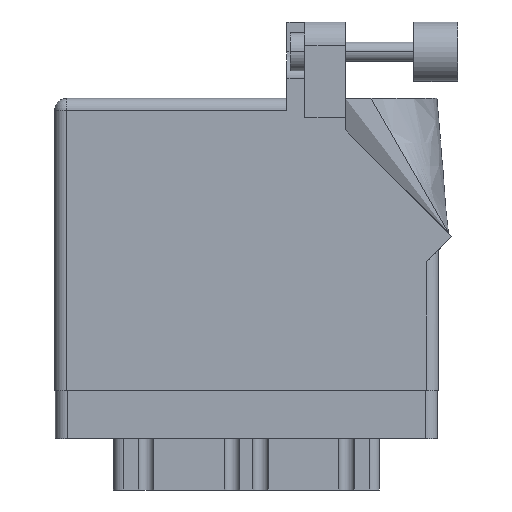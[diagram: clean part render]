
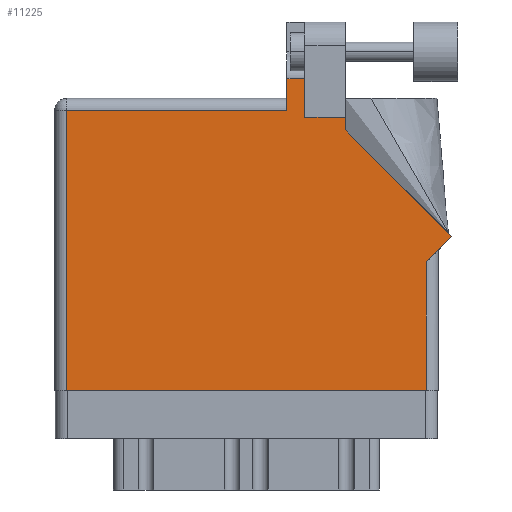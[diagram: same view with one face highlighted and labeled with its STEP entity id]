
A CAD part, front view. The second image highlights one B-rep face of the part: STEP entity #11225.
In plain terms, the highlighted face is planar.
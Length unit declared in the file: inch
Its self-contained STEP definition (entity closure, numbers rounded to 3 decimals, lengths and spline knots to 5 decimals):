
#45 = EDGE_CURVE ( 'NONE', #4962, #10918, #9773, .T. ) ;
#49 = CARTESIAN_POINT ( 'NONE',  ( 1.217, 1.6315, 0. ) ) ;
#969 = LINE ( 'NONE', #33979, #7254 ) ;
#1072 = CARTESIAN_POINT ( 'NONE',  ( 1.217, 1.53, 0. ) ) ;
#1214 = VERTEX_POINT ( 'NONE', #5678 ) ;
#1760 = VERTEX_POINT ( 'NONE', #22241 ) ;
#2330 = VECTOR ( 'NONE', #30479, 39.37008 ) ;
#2416 = VECTOR ( 'NONE', #27783, 39.37008 ) ;
#3102 = LINE ( 'NONE', #29622, #27266 ) ;
#3368 = CARTESIAN_POINT ( 'NONE',  ( 1.524, 1.43, 0. ) ) ;
#4962 = VERTEX_POINT ( 'NONE', #49 ) ;
#5392 = CARTESIAN_POINT ( 'NONE',  ( 1.311, 1.6315, 0. ) ) ;
#5678 = CARTESIAN_POINT ( 'NONE',  ( 1.948, 0.675, 0. ) ) ;
#6646 = EDGE_CURVE ( 'NONE', #15269, #12626, #13773, .T. ) ;
#7254 = VECTOR ( 'NONE', #25110, 39.37008 ) ;
#7283 = CARTESIAN_POINT ( 'NONE',  ( 0., 1.468, 0. ) ) ;
#7368 = VECTOR ( 'NONE', #35777, 39.37008 ) ;
#7680 = LINE ( 'NONE', #7283, #33889 ) ;
#7797 = DIRECTION ( 'NONE',  ( -1., 0., 0. ) ) ;
#7816 = DIRECTION ( 'NONE',  ( 0., 1., 0. ) ) ;
#8453 = VECTOR ( 'NONE', #7816, 39.37008 ) ;
#8519 = LINE ( 'NONE', #21163, #10813 ) ;
#9773 = LINE ( 'NONE', #1072, #2416 ) ;
#10010 = VECTOR ( 'NONE', #32989, 39.37008 ) ;
#10099 = EDGE_CURVE ( 'NONE', #18608, #1214, #24042, .T. ) ;
#10482 = AXIS2_PLACEMENT_3D ( 'NONE', #13750, #14530, #7797 ) ;
#10813 = VECTOR ( 'NONE', #23739, 39.37008 ) ;
#10918 = VERTEX_POINT ( 'NONE', #35880 ) ;
#11225 = ADVANCED_FACE ( 'NONE', ( #35449 ), #22645, .F. ) ;
#11258 = VECTOR ( 'NONE', #38801, 39.37008 ) ;
#11544 = EDGE_LOOP ( 'NONE', ( #30984, #26081, #30827, #28500, #20533, #27481, #18279, #28462, #35621, #21153, #14985 ) ) ;
#12437 = CARTESIAN_POINT ( 'NONE',  ( 1.524, 1.36442, 0. ) ) ;
#12626 = VERTEX_POINT ( 'NONE', #18458 ) ;
#12640 = EDGE_CURVE ( 'NONE', #22661, #18608, #17687, .T. ) ;
#13436 = DIRECTION ( 'NONE',  ( -1., 0., 0. ) ) ;
#13750 = CARTESIAN_POINT ( 'NONE',  ( 0., 1.53, 0. ) ) ;
#13773 = LINE ( 'NONE', #25844, #8453 ) ;
#14530 = DIRECTION ( 'NONE',  ( 0., 0., -1. ) ) ;
#14985 = ORIENTED_EDGE ( 'NONE', *, *, #28324, .T. ) ;
#15187 = DIRECTION ( 'NONE',  ( 0.707, 0.707, 0. ) ) ;
#15269 = VERTEX_POINT ( 'NONE', #12437 ) ;
#17625 = LINE ( 'NONE', #26726, #7368 ) ;
#17687 = LINE ( 'NONE', #18267, #11258 ) ;
#18267 = CARTESIAN_POINT ( 'NONE',  ( 0., 0., 0. ) ) ;
#18279 = ORIENTED_EDGE ( 'NONE', *, *, #10099, .T. ) ;
#18458 = CARTESIAN_POINT ( 'NONE',  ( 1.524, 1.43, 0. ) ) ;
#18608 = VERTEX_POINT ( 'NONE', #37759 ) ;
#19202 = LINE ( 'NONE', #3368, #2330 ) ;
#19732 = EDGE_CURVE ( 'NONE', #1214, #1760, #3102, .T. ) ;
#20533 = ORIENTED_EDGE ( 'NONE', *, *, #34644, .T. ) ;
#21153 = ORIENTED_EDGE ( 'NONE', *, *, #6646, .T. ) ;
#21163 = CARTESIAN_POINT ( 'NONE',  ( 0.062, 0., 0. ) ) ;
#22241 = CARTESIAN_POINT ( 'NONE',  ( 2.08071, 0.80771, 0. ) ) ;
#22645 = PLANE ( 'NONE',  #10482 ) ;
#22661 = VERTEX_POINT ( 'NONE', #27908 ) ;
#23739 = DIRECTION ( 'NONE',  ( 0., -1., 0. ) ) ;
#24042 = LINE ( 'NONE', #36070, #25377 ) ;
#25026 = VERTEX_POINT ( 'NONE', #28873 ) ;
#25110 = DIRECTION ( 'NONE',  ( -0.707, 0.707, 0. ) ) ;
#25377 = VECTOR ( 'NONE', #27594, 39.37008 ) ;
#25844 = CARTESIAN_POINT ( 'NONE',  ( 1.524, 1.36442, 0. ) ) ;
#26081 = ORIENTED_EDGE ( 'NONE', *, *, #35773, .T. ) ;
#26388 = VERTEX_POINT ( 'NONE', #31179 ) ;
#26726 = CARTESIAN_POINT ( 'NONE',  ( 1.64177, 1.6315, 0. ) ) ;
#27266 = VECTOR ( 'NONE', #15187, 39.37008 ) ;
#27481 = ORIENTED_EDGE ( 'NONE', *, *, #12640, .T. ) ;
#27594 = DIRECTION ( 'NONE',  ( 0., 1., 0. ) ) ;
#27783 = DIRECTION ( 'NONE',  ( 0., -1., 0. ) ) ;
#27908 = CARTESIAN_POINT ( 'NONE',  ( 0.062, 0., 0. ) ) ;
#28324 = EDGE_CURVE ( 'NONE', #12626, #26388, #19202, .T. ) ;
#28462 = ORIENTED_EDGE ( 'NONE', *, *, #19732, .T. ) ;
#28500 = ORIENTED_EDGE ( 'NONE', *, *, #31473, .T. ) ;
#28873 = CARTESIAN_POINT ( 'NONE',  ( 0.062, 1.468, 0. ) ) ;
#29298 = EDGE_CURVE ( 'NONE', #1760, #15269, #969, .T. ) ;
#29622 = CARTESIAN_POINT ( 'NONE',  ( 2.01, 0.737, 0. ) ) ;
#30231 = LINE ( 'NONE', #33378, #10010 ) ;
#30479 = DIRECTION ( 'NONE',  ( -1., 0., 0. ) ) ;
#30827 = ORIENTED_EDGE ( 'NONE', *, *, #45, .T. ) ;
#30984 = ORIENTED_EDGE ( 'NONE', *, *, #37310, .T. ) ;
#31179 = CARTESIAN_POINT ( 'NONE',  ( 1.311, 1.43, 0. ) ) ;
#31473 = EDGE_CURVE ( 'NONE', #10918, #25026, #7680, .T. ) ;
#32989 = DIRECTION ( 'NONE',  ( 0., 1., 0. ) ) ;
#33378 = CARTESIAN_POINT ( 'NONE',  ( 1.311, 1.43, 0. ) ) ;
#33889 = VECTOR ( 'NONE', #13436, 39.37008 ) ;
#33979 = CARTESIAN_POINT ( 'NONE',  ( 2.08071, 0.80771, 0. ) ) ;
#34644 = EDGE_CURVE ( 'NONE', #25026, #22661, #8519, .T. ) ;
#35282 = VERTEX_POINT ( 'NONE', #5392 ) ;
#35449 = FACE_OUTER_BOUND ( 'NONE', #11544, .T. ) ;
#35621 = ORIENTED_EDGE ( 'NONE', *, *, #29298, .T. ) ;
#35773 = EDGE_CURVE ( 'NONE', #35282, #4962, #17625, .T. ) ;
#35777 = DIRECTION ( 'NONE',  ( -1., 0., 0. ) ) ;
#35880 = CARTESIAN_POINT ( 'NONE',  ( 1.217, 1.468, 0. ) ) ;
#36070 = CARTESIAN_POINT ( 'NONE',  ( 1.948, 0.737, 0. ) ) ;
#37310 = EDGE_CURVE ( 'NONE', #26388, #35282, #30231, .T. ) ;
#37759 = CARTESIAN_POINT ( 'NONE',  ( 1.948, 0., 0. ) ) ;
#38801 = DIRECTION ( 'NONE',  ( 1., 0., 0. ) ) ;
